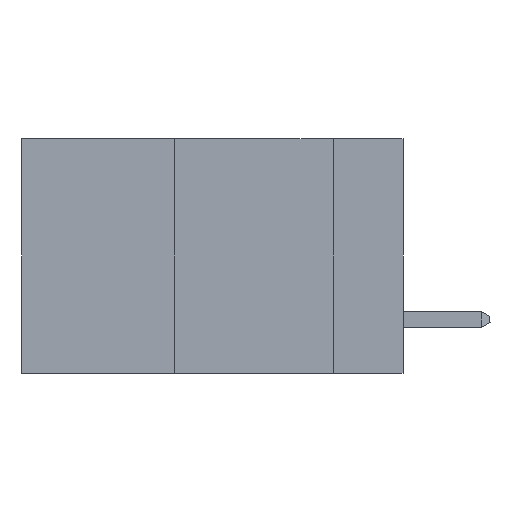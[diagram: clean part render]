
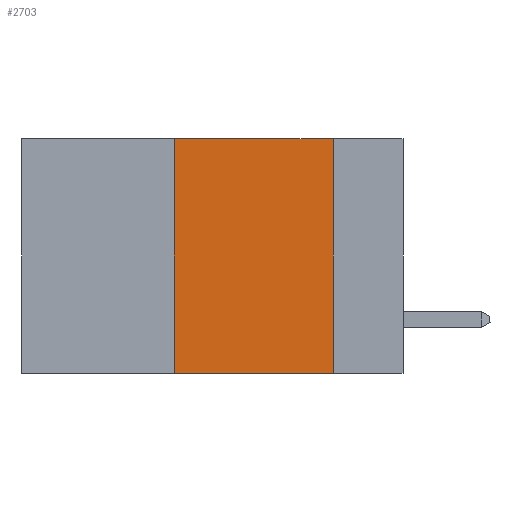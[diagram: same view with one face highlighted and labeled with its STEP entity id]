
A CAD part, left-side view. The second image highlights one B-rep face of the part: STEP entity #2703.
In plain terms, the highlighted planar face has unit normal (-1, 0, 0).
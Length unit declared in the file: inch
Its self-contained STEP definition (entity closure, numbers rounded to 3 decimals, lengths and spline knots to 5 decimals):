
#1758 = ORIENTED_EDGE ( 'NONE', *, *, #15724, .F. ) ;
#1923 = ORIENTED_EDGE ( 'NONE', *, *, #20384, .F. ) ;
#1946 = ORIENTED_EDGE ( 'NONE', *, *, #22388, .T. ) ;
#1964 = VERTEX_POINT ( 'NONE', #19746 ) ;
#2120 = PLANE ( 'NONE',  #13357 ) ;
#2703 = ADVANCED_FACE ( 'NONE', ( #3677 ), #2120, .F. ) ;
#2883 = CARTESIAN_POINT ( 'NONE',  ( 0., 0.11, -0.37 ) ) ;
#3413 = CARTESIAN_POINT ( 'NONE',  ( 0., 0.6, 0. ) ) ;
#3666 = VECTOR ( 'NONE', #13120, 39.37008 ) ;
#3677 = FACE_OUTER_BOUND ( 'NONE', #6431, .T. ) ;
#4756 = CARTESIAN_POINT ( 'NONE',  ( 0., 0.6, -0.37 ) ) ;
#6283 = CARTESIAN_POINT ( 'NONE',  ( 0., 0.6, 0. ) ) ;
#6431 = EDGE_LOOP ( 'NONE', ( #1758, #20107, #1923, #1946 ) ) ;
#7020 = VECTOR ( 'NONE', #12591, 39.37008 ) ;
#7147 = CARTESIAN_POINT ( 'NONE',  ( 0., 0.36, 0. ) ) ;
#7566 = LINE ( 'NONE', #3413, #7020 ) ;
#7712 = LINE ( 'NONE', #10968, #3666 ) ;
#8081 = DIRECTION ( 'NONE',  ( 0., 0., -1. ) ) ;
#8274 = EDGE_CURVE ( 'NONE', #11090, #1964, #7566, .T. ) ;
#8606 = LINE ( 'NONE', #4756, #21751 ) ;
#10614 = VERTEX_POINT ( 'NONE', #17701 ) ;
#10968 = CARTESIAN_POINT ( 'NONE',  ( 0., 0.11, 0. ) ) ;
#11090 = VERTEX_POINT ( 'NONE', #17128 ) ;
#11545 = LINE ( 'NONE', #7147, #20714 ) ;
#12591 = DIRECTION ( 'NONE',  ( 0., -1., 0. ) ) ;
#13120 = DIRECTION ( 'NONE',  ( 0., 0., -1. ) ) ;
#13357 = AXIS2_PLACEMENT_3D ( 'NONE', #6283, #17231, #8081 ) ;
#14019 = DIRECTION ( 'NONE',  ( 0., -1., 0. ) ) ;
#15724 = EDGE_CURVE ( 'NONE', #1964, #18643, #7712, .T. ) ;
#17128 = CARTESIAN_POINT ( 'NONE',  ( 0., 0.36, 0. ) ) ;
#17231 = DIRECTION ( 'NONE',  ( 1., 0., 0. ) ) ;
#17701 = CARTESIAN_POINT ( 'NONE',  ( 0., 0.36, -0.37 ) ) ;
#18643 = VERTEX_POINT ( 'NONE', #2883 ) ;
#19746 = CARTESIAN_POINT ( 'NONE',  ( 0., 0.11, 0. ) ) ;
#20107 = ORIENTED_EDGE ( 'NONE', *, *, #8274, .F. ) ;
#20384 = EDGE_CURVE ( 'NONE', #10614, #11090, #11545, .T. ) ;
#20714 = VECTOR ( 'NONE', #21814, 39.37008 ) ;
#21751 = VECTOR ( 'NONE', #14019, 39.37008 ) ;
#21814 = DIRECTION ( 'NONE',  ( 0., 0., 1. ) ) ;
#22388 = EDGE_CURVE ( 'NONE', #10614, #18643, #8606, .T. ) ;
